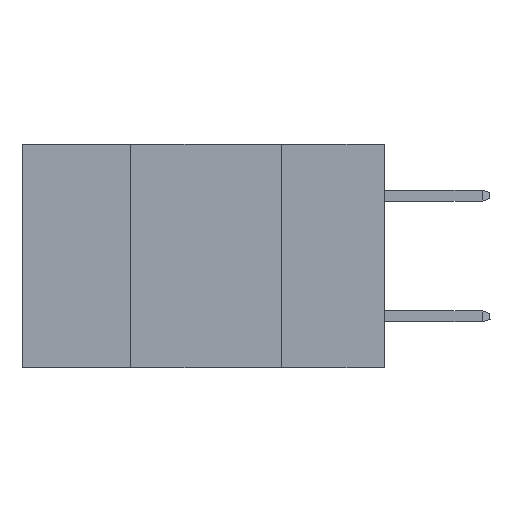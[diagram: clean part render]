
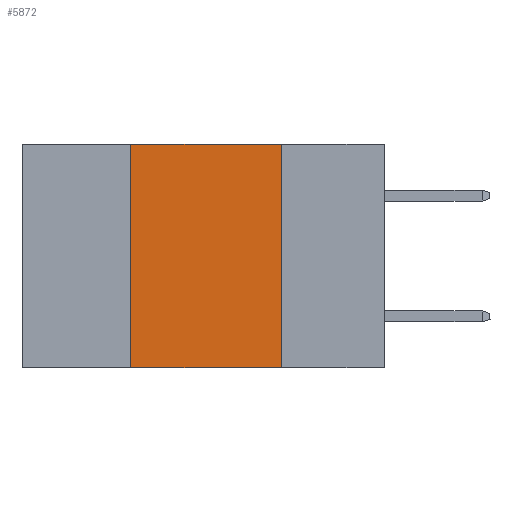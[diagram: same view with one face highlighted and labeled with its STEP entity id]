
A CAD part, left-side view. The second image highlights one B-rep face of the part: STEP entity #5872.
In plain terms, the highlighted planar face has unit normal (-1, 0, 0).
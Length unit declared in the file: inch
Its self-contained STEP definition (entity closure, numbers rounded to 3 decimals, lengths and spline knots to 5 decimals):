
#606 = CARTESIAN_POINT ( 'NONE',  ( 0., 0.17, -0.37 ) ) ;
#901 = ORIENTED_EDGE ( 'NONE', *, *, #6399, .F. ) ;
#933 = DIRECTION ( 'NONE',  ( 0., -1., 0. ) ) ;
#973 = CARTESIAN_POINT ( 'NONE',  ( 0., 0.6, 0. ) ) ;
#1274 = EDGE_CURVE ( 'NONE', #5943, #7871, #11263, .T. ) ;
#1369 = CARTESIAN_POINT ( 'NONE',  ( 0., 0.42, -0.37 ) ) ;
#1581 = DIRECTION ( 'NONE',  ( 0., -1., 0. ) ) ;
#1596 = CARTESIAN_POINT ( 'NONE',  ( 0., 0.6, -0.37 ) ) ;
#2658 = VECTOR ( 'NONE', #5798, 39.37008 ) ;
#2856 = VECTOR ( 'NONE', #5384, 39.37008 ) ;
#2894 = VECTOR ( 'NONE', #933, 39.37008 ) ;
#4228 = VERTEX_POINT ( 'NONE', #11638 ) ;
#4365 = ORIENTED_EDGE ( 'NONE', *, *, #1274, .T. ) ;
#4596 = DIRECTION ( 'NONE',  ( 0., 0., -1. ) ) ;
#4782 = DIRECTION ( 'NONE',  ( 1., 0., 0. ) ) ;
#5384 = DIRECTION ( 'NONE',  ( 0., 0., -1. ) ) ;
#5783 = CARTESIAN_POINT ( 'NONE',  ( 0., 0.42, -0.37 ) ) ;
#5798 = DIRECTION ( 'NONE',  ( 0., 0., 1. ) ) ;
#5872 = ADVANCED_FACE ( 'NONE', ( #15104 ), #6235, .F. ) ;
#5943 = VERTEX_POINT ( 'NONE', #1369 ) ;
#6235 = PLANE ( 'NONE',  #12546 ) ;
#6399 = EDGE_CURVE ( 'NONE', #5943, #14674, #15620, .T. ) ;
#6608 = CARTESIAN_POINT ( 'NONE',  ( 0., 0.42, 0. ) ) ;
#6618 = EDGE_CURVE ( 'NONE', #4228, #7871, #12285, .T. ) ;
#6903 = ORIENTED_EDGE ( 'NONE', *, *, #6618, .F. ) ;
#7427 = CARTESIAN_POINT ( 'NONE',  ( 0., 0.17, -0.37 ) ) ;
#7871 = VERTEX_POINT ( 'NONE', #7427 ) ;
#8708 = CARTESIAN_POINT ( 'NONE',  ( 0., 0.6, 0. ) ) ;
#8880 = EDGE_CURVE ( 'NONE', #14674, #4228, #9890, .T. ) ;
#9890 = LINE ( 'NONE', #973, #2894 ) ;
#10157 = ORIENTED_EDGE ( 'NONE', *, *, #8880, .F. ) ;
#11263 = LINE ( 'NONE', #1596, #14427 ) ;
#11638 = CARTESIAN_POINT ( 'NONE',  ( 0., 0.17, 0. ) ) ;
#12285 = LINE ( 'NONE', #606, #2856 ) ;
#12546 = AXIS2_PLACEMENT_3D ( 'NONE', #8708, #4782, #4596 ) ;
#14427 = VECTOR ( 'NONE', #1581, 39.37008 ) ;
#14674 = VERTEX_POINT ( 'NONE', #6608 ) ;
#15104 = FACE_OUTER_BOUND ( 'NONE', #15878, .T. ) ;
#15620 = LINE ( 'NONE', #5783, #2658 ) ;
#15878 = EDGE_LOOP ( 'NONE', ( #6903, #10157, #901, #4365 ) ) ;
